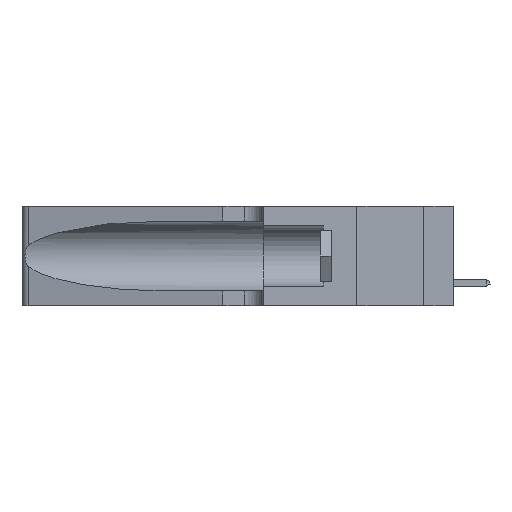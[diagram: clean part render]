
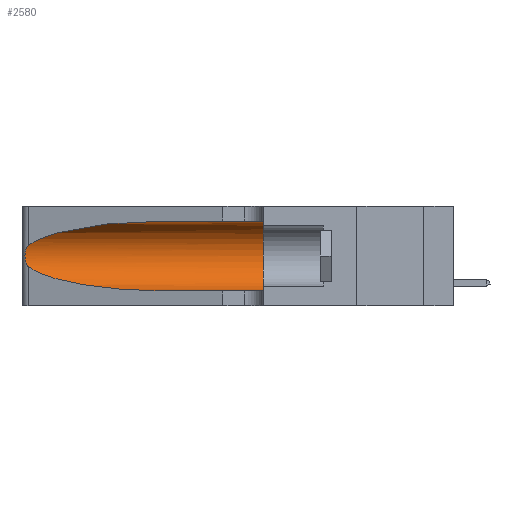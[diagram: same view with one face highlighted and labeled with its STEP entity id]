
A CAD part, left-side view. The second image highlights one B-rep face of the part: STEP entity #2580.
In plain terms, the highlighted cylindrical face has radius 3.308 mm (diameter 6.617 mm), a partial arc.
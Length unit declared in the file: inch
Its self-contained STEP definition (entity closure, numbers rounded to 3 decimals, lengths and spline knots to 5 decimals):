
#58 = VECTOR ( 'NONE', #9530, 39.37008 ) ;
#546 = VERTEX_POINT ( 'NONE', #18041 ) ;
#1122 = CARTESIAN_POINT ( 'NONE',  ( 0.25854, 1.2359, 0.20912 ) ) ;
#1262 = CARTESIAN_POINT ( 'NONE',  ( 0.25487, 1.22718, 0.22369 ) ) ;
#1314 = EDGE_CURVE ( 'NONE', #4869, #15549, #3938, .T. ) ;
#1337 = CARTESIAN_POINT ( 'NONE',  ( 0.25487, 1.22718, 0.14631 ) ) ;
#1563 = LINE ( 'NONE', #10648, #4076 ) ;
#2580 = ADVANCED_FACE ( 'NONE', ( #14815 ), #10516, .F. ) ;
#2763 = CARTESIAN_POINT ( 'NONE',  ( 0.2373, 1.15595, 0.08982 ) ) ;
#2884 = CARTESIAN_POINT ( 'NONE',  ( 0.25856, 1.23593, 0.16098 ) ) ;
#3254 = VERTEX_POINT ( 'NONE', #16070 ) ;
#3510 =( BOUNDED_CURVE ( )  B_SPLINE_CURVE ( 3, ( #18875, #2763, #12468, #14101 ),
 .UNSPECIFIED., .F., .F. ) 
 B_SPLINE_CURVE_WITH_KNOTS ( ( 4, 4 ),
 ( 3.44316, 4.71239 ),
 .UNSPECIFIED. ) 
 CURVE ( )  GEOMETRIC_REPRESENTATION_ITEM ( )  RATIONAL_B_SPLINE_CURVE ( ( 1., 0.87, 0.87, 1. ) ) 
 REPRESENTATION_ITEM ( '' )  );
#3617 = AXIS2_PLACEMENT_3D ( 'NONE', #7141, #9094, #15671 ) ;
#3938 = CIRCLE ( 'NONE', #3617, 0.13025 ) ;
#4076 = VECTOR ( 'NONE', #19029, 39.37008 ) ;
#4286 = CARTESIAN_POINT ( 'NONE',  ( 0.26017, 1.23833, 0.17102 ) ) ;
#4572 = CARTESIAN_POINT ( 'NONE',  ( 0.26075, 1.23896, 0.19203 ) ) ;
#4850 = LINE ( 'NONE', #6949, #58 ) ;
#4869 = VERTEX_POINT ( 'NONE', #9767 ) ;
#5374 = ORIENTED_EDGE ( 'NONE', *, *, #7685, .T. ) ;
#6136 = CARTESIAN_POINT ( 'NONE',  ( 0.25639, 1.23184, 0.21858 ) ) ;
#6949 = CARTESIAN_POINT ( 'NONE',  ( 0.1305, 1.61858, 0.05475 ) ) ;
#7141 = CARTESIAN_POINT ( 'NONE',  ( 0.1305, 0.35, 0.185 ) ) ;
#7685 = EDGE_CURVE ( 'NONE', #11835, #546, #19187, .T. ) ;
#7695 = CARTESIAN_POINT ( 'NONE',  ( 0.25787, 1.23484, 0.2124 ) ) ;
#7831 = ORIENTED_EDGE ( 'NONE', *, *, #11229, .T. ) ;
#9094 = DIRECTION ( 'NONE',  ( 0., 1., 0. ) ) ;
#9530 = DIRECTION ( 'NONE',  ( 0., -1., 0. ) ) ;
#9546 = ORIENTED_EDGE ( 'NONE', *, *, #15308, .F. ) ;
#9767 = CARTESIAN_POINT ( 'NONE',  ( 0.1305, 0.35, 0.31525 ) ) ;
#10516 = CYLINDRICAL_SURFACE ( 'NONE', #19261, 0.13025 ) ;
#10648 = CARTESIAN_POINT ( 'NONE',  ( 0.1305, 1.61858, 0.31525 ) ) ;
#10744 = CARTESIAN_POINT ( 'NONE',  ( 0.25487, 1.22718, 0.14631 ) ) ;
#10920 = CARTESIAN_POINT ( 'NONE',  ( 0.26075, 1.23896, 0.178 ) ) ;
#11229 = EDGE_CURVE ( 'NONE', #546, #14526, #13209, .T. ) ;
#11639 = ORIENTED_EDGE ( 'NONE', *, *, #19614, .T. ) ;
#11835 = VERTEX_POINT ( 'NONE', #13541 ) ;
#12141 = EDGE_LOOP ( 'NONE', ( #5374, #7831, #11639, #18577, #14129, #9546 ) ) ;
#12459 = CARTESIAN_POINT ( 'NONE',  ( 0.25789, 1.23486, 0.15765 ) ) ;
#12468 = CARTESIAN_POINT ( 'NONE',  ( 0.18966, 0.96281, 0.05475 ) ) ;
#12844 = CARTESIAN_POINT ( 'NONE',  ( 0.2373, 1.15595, 0.28018 ) ) ;
#13209 = B_SPLINE_CURVE_WITH_KNOTS ( 'NONE', 3,
 ( #1262, #17457, #6136, #7695, #1122, #17385, #4572, #10920, #4286, #2884, #12459, #20419, #18992, #1337 ),
 .UNSPECIFIED., .F., .F.,
 ( 4, 2, 2, 2, 2, 2, 4 ),
 ( 0., 0.00027, 0.00053, 0.00107, 0.0016, 0.00187, 0.00214 ),
 .UNSPECIFIED. ) ;
#13541 = CARTESIAN_POINT ( 'NONE',  ( 0.1305, 0.72297, 0.31525 ) ) ;
#14057 = CARTESIAN_POINT ( 'NONE',  ( 0.1305, 0.72297, 0.31525 ) ) ;
#14100 = DIRECTION ( 'NONE',  ( 0., -1., 0. ) ) ;
#14101 = CARTESIAN_POINT ( 'NONE',  ( 0.1305, 0.72297, 0.05475 ) ) ;
#14129 = ORIENTED_EDGE ( 'NONE', *, *, #1314, .F. ) ;
#14526 = VERTEX_POINT ( 'NONE', #10744 ) ;
#14815 = FACE_OUTER_BOUND ( 'NONE', #12141, .T. ) ;
#15308 = EDGE_CURVE ( 'NONE', #11835, #4869, #1563, .T. ) ;
#15549 = VERTEX_POINT ( 'NONE', #20273 ) ;
#15671 = DIRECTION ( 'NONE',  ( 0., 0., 1. ) ) ;
#16070 = CARTESIAN_POINT ( 'NONE',  ( 0.1305, 0.72297, 0.05475 ) ) ;
#17385 = CARTESIAN_POINT ( 'NONE',  ( 0.26018, 1.23835, 0.19895 ) ) ;
#17457 = CARTESIAN_POINT ( 'NONE',  ( 0.25555, 1.22994, 0.2215 ) ) ;
#18041 = CARTESIAN_POINT ( 'NONE',  ( 0.25487, 1.22718, 0.22369 ) ) ;
#18577 = ORIENTED_EDGE ( 'NONE', *, *, #20877, .T. ) ;
#18875 = CARTESIAN_POINT ( 'NONE',  ( 0.25487, 1.22718, 0.14631 ) ) ;
#18959 = CARTESIAN_POINT ( 'NONE',  ( 0.18966, 0.96281, 0.31525 ) ) ;
#18992 = CARTESIAN_POINT ( 'NONE',  ( 0.25555, 1.22993, 0.14849 ) ) ;
#19029 = DIRECTION ( 'NONE',  ( 0., -1., 0. ) ) ;
#19068 = DIRECTION ( 'NONE',  ( 0., 0., -1. ) ) ;
#19187 =( BOUNDED_CURVE ( )  B_SPLINE_CURVE ( 3, ( #14057, #18959, #12844, #20822 ),
 .UNSPECIFIED., .F., .T. ) 
 B_SPLINE_CURVE_WITH_KNOTS ( ( 4, 4 ),
 ( 1.5708, 2.84003 ),
 .UNSPECIFIED. ) 
 CURVE ( )  GEOMETRIC_REPRESENTATION_ITEM ( )  RATIONAL_B_SPLINE_CURVE ( ( 1., 0.87, 0.87, 1. ) ) 
 REPRESENTATION_ITEM ( '' )  );
#19261 = AXIS2_PLACEMENT_3D ( 'NONE', #20795, #14100, #19068 ) ;
#19614 = EDGE_CURVE ( 'NONE', #14526, #3254, #3510, .T. ) ;
#20273 = CARTESIAN_POINT ( 'NONE',  ( 0.1305, 0.35, 0.05475 ) ) ;
#20419 = CARTESIAN_POINT ( 'NONE',  ( 0.25639, 1.23186, 0.15144 ) ) ;
#20795 = CARTESIAN_POINT ( 'NONE',  ( 0.1305, 1.61858, 0.185 ) ) ;
#20822 = CARTESIAN_POINT ( 'NONE',  ( 0.25487, 1.22718, 0.22369 ) ) ;
#20877 = EDGE_CURVE ( 'NONE', #3254, #15549, #4850, .T. ) ;
